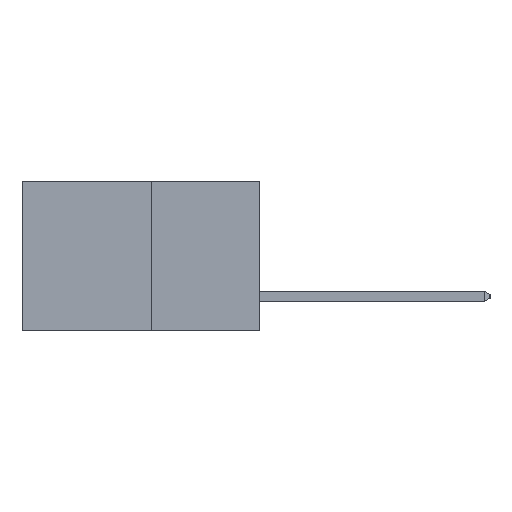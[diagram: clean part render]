
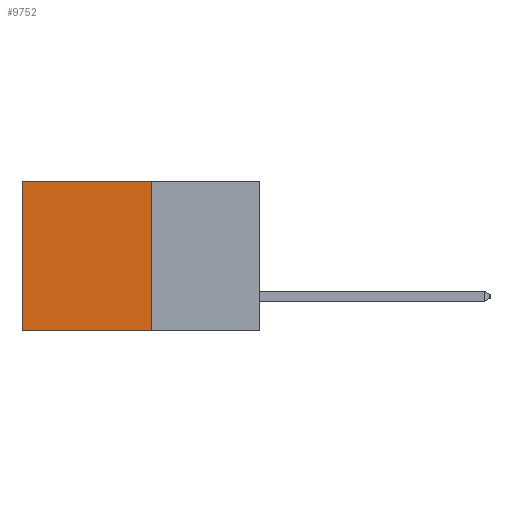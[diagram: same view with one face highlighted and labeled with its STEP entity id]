
A CAD part, left-side view. The second image highlights one B-rep face of the part: STEP entity #9752.
In plain terms, the highlighted planar face has unit normal (-1, 0, 0).
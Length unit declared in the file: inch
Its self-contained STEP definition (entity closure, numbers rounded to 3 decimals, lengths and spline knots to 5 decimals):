
#145 = VERTEX_POINT ( 'NONE', #7862 ) ;
#849 = CARTESIAN_POINT ( 'NONE',  ( 0.277, 0.27, -0.37 ) ) ;
#1138 = EDGE_CURVE ( 'NONE', #6827, #10851, #9963, .T. ) ;
#1317 = ORIENTED_EDGE ( 'NONE', *, *, #9606, .F. ) ;
#1406 = CARTESIAN_POINT ( 'NONE',  ( 0.277, 0.59, 0. ) ) ;
#1524 = CARTESIAN_POINT ( 'NONE',  ( 0.277, 0.59, -0.37 ) ) ;
#1773 = ORIENTED_EDGE ( 'NONE', *, *, #1138, .F. ) ;
#2120 = CARTESIAN_POINT ( 'NONE',  ( 0.277, 0.27, -0.37 ) ) ;
#2332 = EDGE_CURVE ( 'NONE', #5905, #10851, #7474, .T. ) ;
#2368 = CARTESIAN_POINT ( 'NONE',  ( 0.277, 0.27, -0.37 ) ) ;
#2957 = VECTOR ( 'NONE', #5020, 39.37008 ) ;
#3408 = CARTESIAN_POINT ( 'NONE',  ( 0.277, 0.59, -0.37 ) ) ;
#3416 = LINE ( 'NONE', #9439, #5527 ) ;
#3724 = DIRECTION ( 'NONE',  ( 1., 0., 0. ) ) ;
#4248 = ORIENTED_EDGE ( 'NONE', *, *, #8157, .T. ) ;
#5020 = DIRECTION ( 'NONE',  ( 0., 0., -1. ) ) ;
#5128 = DIRECTION ( 'NONE',  ( 0., 0., -1. ) ) ;
#5482 = VECTOR ( 'NONE', #9046, 39.37008 ) ;
#5527 = VECTOR ( 'NONE', #10299, 39.37008 ) ;
#5636 = EDGE_LOOP ( 'NONE', ( #11068, #1773, #1317, #4248 ) ) ;
#5905 = VERTEX_POINT ( 'NONE', #1406 ) ;
#6827 = VERTEX_POINT ( 'NONE', #2120 ) ;
#7076 = FACE_OUTER_BOUND ( 'NONE', #5636, .T. ) ;
#7474 = LINE ( 'NONE', #1524, #2957 ) ;
#7862 = CARTESIAN_POINT ( 'NONE',  ( 0.277, 0.27, 0. ) ) ;
#8062 = AXIS2_PLACEMENT_3D ( 'NONE', #849, #3724, #9969 ) ;
#8157 = EDGE_CURVE ( 'NONE', #145, #5905, #3416, .T. ) ;
#8787 = VECTOR ( 'NONE', #5128, 39.37008 ) ;
#8963 = CARTESIAN_POINT ( 'NONE',  ( 0.277, 0.27, -0.37 ) ) ;
#9046 = DIRECTION ( 'NONE',  ( 0., 1., 0. ) ) ;
#9106 = PLANE ( 'NONE',  #8062 ) ;
#9439 = CARTESIAN_POINT ( 'NONE',  ( 0.277, 0.27, 0. ) ) ;
#9606 = EDGE_CURVE ( 'NONE', #145, #6827, #11398, .T. ) ;
#9752 = ADVANCED_FACE ( 'NONE', ( #7076 ), #9106, .F. ) ;
#9963 = LINE ( 'NONE', #8963, #5482 ) ;
#9969 = DIRECTION ( 'NONE',  ( 0., 0., -1. ) ) ;
#10299 = DIRECTION ( 'NONE',  ( 0., 1., 0. ) ) ;
#10851 = VERTEX_POINT ( 'NONE', #3408 ) ;
#11068 = ORIENTED_EDGE ( 'NONE', *, *, #2332, .T. ) ;
#11398 = LINE ( 'NONE', #2368, #8787 ) ;
